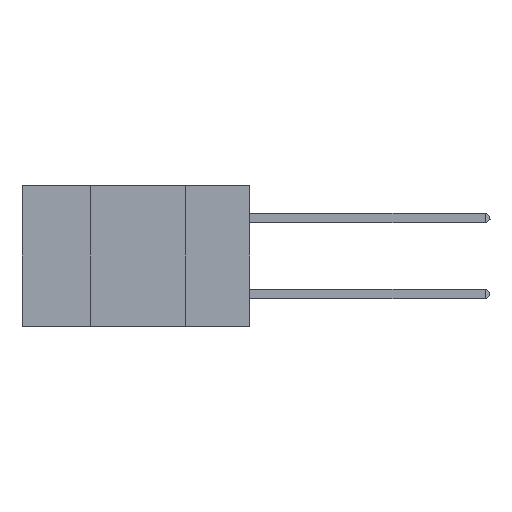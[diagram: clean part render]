
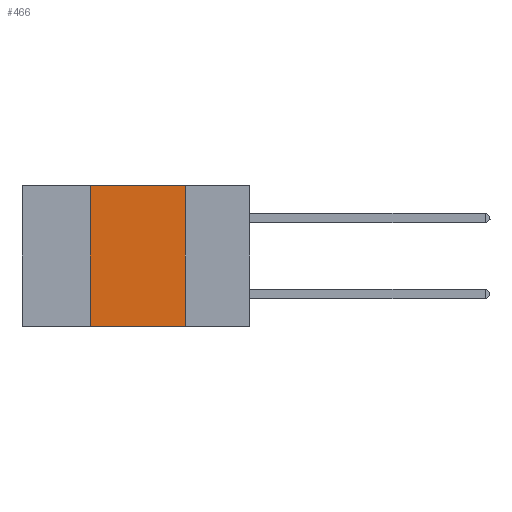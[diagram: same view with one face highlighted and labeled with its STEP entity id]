
A CAD part, left-side view. The second image highlights one B-rep face of the part: STEP entity #466.
In plain terms, the highlighted planar face has unit normal (-1, 0, 0).
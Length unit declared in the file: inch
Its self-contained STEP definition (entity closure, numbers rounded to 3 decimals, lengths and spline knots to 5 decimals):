
#466 = ADVANCED_FACE ( 'NONE', ( #6697 ), #4927, .F. ) ;
#1117 = VECTOR ( 'NONE', #13532, 39.37008 ) ;
#3331 = VERTEX_POINT ( 'NONE', #9632 ) ;
#3902 = ORIENTED_EDGE ( 'NONE', *, *, #15626, .F. ) ;
#3920 = EDGE_CURVE ( 'NONE', #3331, #16449, #20441, .T. ) ;
#4254 = CARTESIAN_POINT ( 'NONE',  ( 0., 0.17, 0. ) ) ;
#4586 = CARTESIAN_POINT ( 'NONE',  ( 0., 0.6, 0. ) ) ;
#4927 = PLANE ( 'NONE',  #9292 ) ;
#5467 = EDGE_LOOP ( 'NONE', ( #21590, #13677, #3902, #10088 ) ) ;
#5786 = VECTOR ( 'NONE', #18678, 39.37008 ) ;
#6012 = EDGE_CURVE ( 'NONE', #15772, #16449, #21068, .T. ) ;
#6697 = FACE_OUTER_BOUND ( 'NONE', #5467, .T. ) ;
#7144 = CARTESIAN_POINT ( 'NONE',  ( 0., 0.17, -0.37 ) ) ;
#8460 = DIRECTION ( 'NONE',  ( 0., 0., 1. ) ) ;
#8569 = CARTESIAN_POINT ( 'NONE',  ( 0., 0.42, 0. ) ) ;
#9292 = AXIS2_PLACEMENT_3D ( 'NONE', #4586, #14774, #20183 ) ;
#9632 = CARTESIAN_POINT ( 'NONE',  ( 0., 0.42, -0.37 ) ) ;
#10088 = ORIENTED_EDGE ( 'NONE', *, *, #3920, .T. ) ;
#10304 = CARTESIAN_POINT ( 'NONE',  ( 0., 0.42, 0. ) ) ;
#11882 = VECTOR ( 'NONE', #8460, 39.37008 ) ;
#13532 = DIRECTION ( 'NONE',  ( 0., -1., 0. ) ) ;
#13551 = LINE ( 'NONE', #8569, #11882 ) ;
#13677 = ORIENTED_EDGE ( 'NONE', *, *, #21144, .F. ) ;
#13826 = VERTEX_POINT ( 'NONE', #10304 ) ;
#13993 = DIRECTION ( 'NONE',  ( 0., 0., -1. ) ) ;
#14774 = DIRECTION ( 'NONE',  ( 1., 0., 0. ) ) ;
#15184 = CARTESIAN_POINT ( 'NONE',  ( 0., 0.6, 0. ) ) ;
#15626 = EDGE_CURVE ( 'NONE', #3331, #13826, #13551, .T. ) ;
#15772 = VERTEX_POINT ( 'NONE', #20933 ) ;
#16449 = VERTEX_POINT ( 'NONE', #7144 ) ;
#17069 = LINE ( 'NONE', #15184, #1117 ) ;
#17235 = CARTESIAN_POINT ( 'NONE',  ( 0., 0.6, -0.37 ) ) ;
#18678 = DIRECTION ( 'NONE',  ( 0., -1., 0. ) ) ;
#20183 = DIRECTION ( 'NONE',  ( 0., 0., -1. ) ) ;
#20361 = VECTOR ( 'NONE', #13993, 39.37008 ) ;
#20441 = LINE ( 'NONE', #17235, #5786 ) ;
#20933 = CARTESIAN_POINT ( 'NONE',  ( 0., 0.17, 0. ) ) ;
#21068 = LINE ( 'NONE', #4254, #20361 ) ;
#21144 = EDGE_CURVE ( 'NONE', #13826, #15772, #17069, .T. ) ;
#21590 = ORIENTED_EDGE ( 'NONE', *, *, #6012, .F. ) ;
